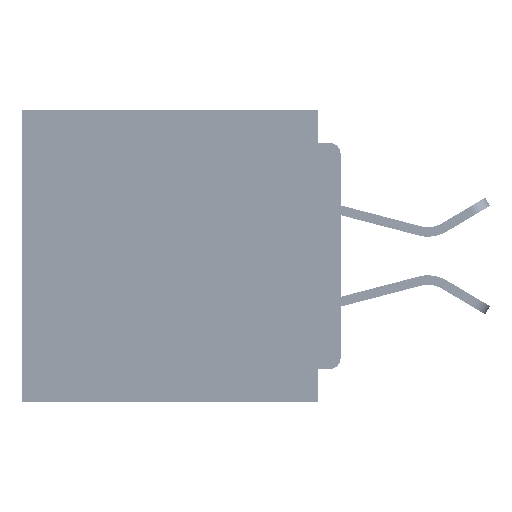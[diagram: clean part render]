
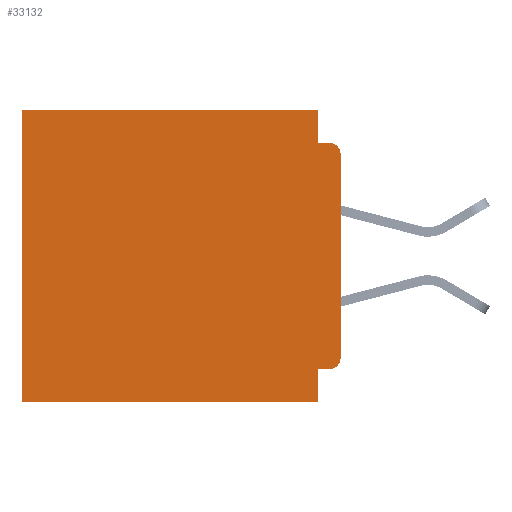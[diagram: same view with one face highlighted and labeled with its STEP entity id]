
A CAD part, left-side view. The second image highlights one B-rep face of the part: STEP entity #33132.
In plain terms, the highlighted planar face has unit normal (-1, 0, 0).
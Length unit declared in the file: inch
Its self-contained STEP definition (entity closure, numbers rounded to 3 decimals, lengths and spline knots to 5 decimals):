
#28 = VECTOR ( 'NONE', #27760, 39.37008 ) ;
#363 = CARTESIAN_POINT ( 'NONE',  ( 0.3, 0.031, -0.045 ) ) ;
#579 = ORIENTED_EDGE ( 'NONE', *, *, #29067, .T. ) ;
#1495 = DIRECTION ( 'NONE',  ( 0., 0., -1. ) ) ;
#2300 = CARTESIAN_POINT ( 'NONE',  ( 0.3, 0., -0.34 ) ) ;
#3067 = AXIS2_PLACEMENT_3D ( 'NONE', #13701, #40624, #17634 ) ;
#3953 = CARTESIAN_POINT ( 'NONE',  ( 0.3, 0., -0.355 ) ) ;
#4730 = CIRCLE ( 'NONE', #33153, 0.015 ) ;
#6853 = ORIENTED_EDGE ( 'NONE', *, *, #9128, .F. ) ;
#7494 = ORIENTED_EDGE ( 'NONE', *, *, #28152, .F. ) ;
#8313 = EDGE_CURVE ( 'NONE', #34130, #39022, #10615, .T. ) ;
#9128 = EDGE_CURVE ( 'NONE', #38181, #34130, #25600, .T. ) ;
#10615 = LINE ( 'NONE', #16313, #22110 ) ;
#10916 = VECTOR ( 'NONE', #35105, 39.37008 ) ;
#11025 = DIRECTION ( 'NONE',  ( 0., 0., -1. ) ) ;
#11883 = EDGE_CURVE ( 'NONE', #48745, #39022, #4730, .T. ) ;
#11983 = LINE ( 'NONE', #3953, #41437 ) ;
#12327 = ORIENTED_EDGE ( 'NONE', *, *, #36677, .F. ) ;
#12462 = VERTEX_POINT ( 'NONE', #2300 ) ;
#12935 = ORIENTED_EDGE ( 'NONE', *, *, #15776, .T. ) ;
#13701 = CARTESIAN_POINT ( 'NONE',  ( 0.3, 0., -0.4 ) ) ;
#14800 = DIRECTION ( 'NONE',  ( 0., 0., -1. ) ) ;
#15776 = EDGE_CURVE ( 'NONE', #38181, #20526, #21193, .T. ) ;
#16313 = CARTESIAN_POINT ( 'NONE',  ( 0.3, 0., -0.045 ) ) ;
#17081 = EDGE_CURVE ( 'NONE', #26061, #48380, #11983, .T. ) ;
#17305 = CARTESIAN_POINT ( 'NONE',  ( 0.3, 0.437, 0. ) ) ;
#17590 = EDGE_CURVE ( 'NONE', #39746, #47358, #49208, .T. ) ;
#17634 = DIRECTION ( 'NONE',  ( 0., 0., -1. ) ) ;
#17639 = DIRECTION ( 'NONE',  ( -1., 0., 0. ) ) ;
#20526 = VERTEX_POINT ( 'NONE', #17305 ) ;
#21193 = LINE ( 'NONE', #46514, #10916 ) ;
#21546 = CARTESIAN_POINT ( 'NONE',  ( 0.3, 0.437, -0.4 ) ) ;
#21757 = CARTESIAN_POINT ( 'NONE',  ( 0.3, 0.015, -0.34 ) ) ;
#21885 = LINE ( 'NONE', #46874, #28 ) ;
#22110 = VECTOR ( 'NONE', #39336, 39.37008 ) ;
#22428 = LINE ( 'NONE', #34118, #32603 ) ;
#23283 = DIRECTION ( 'NONE',  ( 0., 1., 0. ) ) ;
#23298 = CARTESIAN_POINT ( 'NONE',  ( 0.3, 0.015, -0.045 ) ) ;
#23840 = AXIS2_PLACEMENT_3D ( 'NONE', #21757, #48580, #25587 ) ;
#24430 = VECTOR ( 'NONE', #1495, 39.37008 ) ;
#24673 = CARTESIAN_POINT ( 'NONE',  ( 0.3, 0.031, 0. ) ) ;
#25587 = DIRECTION ( 'NONE',  ( 0., 0., -1. ) ) ;
#25600 = LINE ( 'NONE', #24673, #24430 ) ;
#26027 = CARTESIAN_POINT ( 'NONE',  ( 0.3, 0.015, -0.355 ) ) ;
#26061 = VERTEX_POINT ( 'NONE', #26027 ) ;
#27760 = DIRECTION ( 'NONE',  ( 0., 0., -1. ) ) ;
#28152 = EDGE_CURVE ( 'NONE', #48380, #39746, #21885, .T. ) ;
#29067 = EDGE_CURVE ( 'NONE', #20526, #47358, #31434, .T. ) ;
#29624 = ORIENTED_EDGE ( 'NONE', *, *, #17590, .F. ) ;
#31434 = LINE ( 'NONE', #49329, #49446 ) ;
#32603 = VECTOR ( 'NONE', #14800, 39.37008 ) ;
#33132 = ADVANCED_FACE ( 'NONE', ( #36592 ), #48169, .F. ) ;
#33153 = AXIS2_PLACEMENT_3D ( 'NONE', #40628, #17639, #44437 ) ;
#33243 = CARTESIAN_POINT ( 'NONE',  ( 0.3, 0., -0.06 ) ) ;
#33378 = ORIENTED_EDGE ( 'NONE', *, *, #17081, .F. ) ;
#34118 = CARTESIAN_POINT ( 'NONE',  ( 0.3, 0., -0.4 ) ) ;
#34130 = VERTEX_POINT ( 'NONE', #363 ) ;
#34985 = CIRCLE ( 'NONE', #23840, 0.015 ) ;
#35008 = ORIENTED_EDGE ( 'NONE', *, *, #8313, .F. ) ;
#35105 = DIRECTION ( 'NONE',  ( 0., 1., 0. ) ) ;
#35942 = CARTESIAN_POINT ( 'NONE',  ( 0.3, 0.031, -0.4 ) ) ;
#36592 = FACE_OUTER_BOUND ( 'NONE', #47278, .T. ) ;
#36677 = EDGE_CURVE ( 'NONE', #48745, #12462, #22428, .T. ) ;
#36768 = ORIENTED_EDGE ( 'NONE', *, *, #11883, .T. ) ;
#38181 = VERTEX_POINT ( 'NONE', #47063 ) ;
#38296 = CARTESIAN_POINT ( 'NONE',  ( 0.3, 0., -0.4 ) ) ;
#39022 = VERTEX_POINT ( 'NONE', #23298 ) ;
#39336 = DIRECTION ( 'NONE',  ( 0., -1., 0. ) ) ;
#39746 = VERTEX_POINT ( 'NONE', #35942 ) ;
#40211 = VECTOR ( 'NONE', #45837, 39.37008 ) ;
#40624 = DIRECTION ( 'NONE',  ( 1., 0., 0. ) ) ;
#40628 = CARTESIAN_POINT ( 'NONE',  ( 0.3, 0.015, -0.06 ) ) ;
#41437 = VECTOR ( 'NONE', #23283, 39.37008 ) ;
#42009 = CARTESIAN_POINT ( 'NONE',  ( 0.3, 0.031, -0.355 ) ) ;
#42227 = ORIENTED_EDGE ( 'NONE', *, *, #43738, .T. ) ;
#43738 = EDGE_CURVE ( 'NONE', #26061, #12462, #34985, .T. ) ;
#44437 = DIRECTION ( 'NONE',  ( 0., 0., -1. ) ) ;
#45837 = DIRECTION ( 'NONE',  ( 0., 1., 0. ) ) ;
#46514 = CARTESIAN_POINT ( 'NONE',  ( 0.3, 0., 0. ) ) ;
#46874 = CARTESIAN_POINT ( 'NONE',  ( 0.3, 0.031, -0.4 ) ) ;
#47063 = CARTESIAN_POINT ( 'NONE',  ( 0.3, 0.031, 0. ) ) ;
#47278 = EDGE_LOOP ( 'NONE', ( #12327, #36768, #35008, #6853, #12935, #579, #29624, #7494, #33378, #42227 ) ) ;
#47358 = VERTEX_POINT ( 'NONE', #21546 ) ;
#48169 = PLANE ( 'NONE',  #3067 ) ;
#48380 = VERTEX_POINT ( 'NONE', #42009 ) ;
#48580 = DIRECTION ( 'NONE',  ( -1., 0., 0. ) ) ;
#48745 = VERTEX_POINT ( 'NONE', #33243 ) ;
#49208 = LINE ( 'NONE', #38296, #40211 ) ;
#49329 = CARTESIAN_POINT ( 'NONE',  ( 0.3, 0.437, -0.4 ) ) ;
#49446 = VECTOR ( 'NONE', #11025, 39.37008 ) ;
